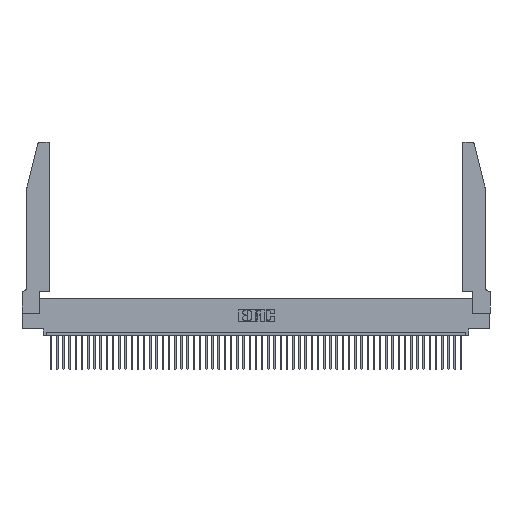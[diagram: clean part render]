
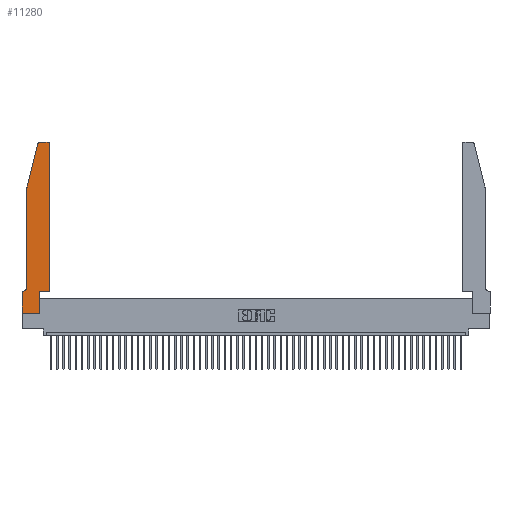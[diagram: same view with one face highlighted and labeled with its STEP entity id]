
A CAD part, top view. The second image highlights one B-rep face of the part: STEP entity #11280.
In plain terms, the highlighted planar face has unit normal (0, 0, 1).
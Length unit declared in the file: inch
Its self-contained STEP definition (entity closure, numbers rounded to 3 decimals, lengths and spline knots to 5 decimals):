
#703 = DIRECTION ( 'NONE',  ( -1., 0., 0. ) ) ;
#1174 = CARTESIAN_POINT ( 'NONE',  ( 0., 0., 0.37 ) ) ;
#1199 = DIRECTION ( 'NONE',  ( 0., 0., 1. ) ) ;
#2062 = CARTESIAN_POINT ( 'NONE',  ( 0.4205, 2.75, 0.37 ) ) ;
#2794 = DIRECTION ( 'NONE',  ( 0., 0., -1. ) ) ;
#3361 = LINE ( 'NONE', #31498, #33414 ) ;
#3362 = CARTESIAN_POINT ( 'NONE',  ( 0.0755, 0.42, 0.37 ) ) ;
#5062 = CARTESIAN_POINT ( 'NONE',  ( 0.0755, 0.35, 0.37 ) ) ;
#5239 = AXIS2_PLACEMENT_3D ( 'NONE', #48911, #1199, #17721 ) ;
#5340 = CARTESIAN_POINT ( 'NONE',  ( 0.2865, 0., 0.37 ) ) ;
#5935 = EDGE_CURVE ( 'NONE', #38857, #20977, #15634, .T. ) ;
#5965 = VECTOR ( 'NONE', #21502, 39.37008 ) ;
#6009 = VERTEX_POINT ( 'NONE', #2062 ) ;
#6143 = CARTESIAN_POINT ( 'NONE',  ( 0.4505, 0.35, 0.37 ) ) ;
#6474 = ORIENTED_EDGE ( 'NONE', *, *, #27926, .T. ) ;
#6939 = EDGE_CURVE ( 'NONE', #16477, #45572, #27984, .T. ) ;
#7575 = LINE ( 'NONE', #18554, #35811 ) ;
#8052 = AXIS2_PLACEMENT_3D ( 'NONE', #14729, #2794, #30981 ) ;
#8343 = ORIENTED_EDGE ( 'NONE', *, *, #14810, .T. ) ;
#8466 = VECTOR ( 'NONE', #29494, 39.37008 ) ;
#9025 = LINE ( 'NONE', #36225, #33503 ) ;
#9367 = ORIENTED_EDGE ( 'NONE', *, *, #30261, .T. ) ;
#9825 = VECTOR ( 'NONE', #703, 39.37008 ) ;
#9875 = DIRECTION ( 'NONE',  ( -0.239, -0.971, 0. ) ) ;
#11235 = EDGE_CURVE ( 'NONE', #22275, #40894, #43234, .T. ) ;
#11280 = ADVANCED_FACE ( 'NONE', ( #45057 ), #34998, .T. ) ;
#11444 = DIRECTION ( 'NONE',  ( 1., 0., 0. ) ) ;
#12366 = VECTOR ( 'NONE', #26677, 39.37008 ) ;
#12925 = ORIENTED_EDGE ( 'NONE', *, *, #33495, .T. ) ;
#13820 = CARTESIAN_POINT ( 'NONE',  ( 0.25487, 2.72718, 0.37 ) ) ;
#14729 = CARTESIAN_POINT ( 'NONE',  ( 0.0055, 0.42, 0.37 ) ) ;
#14810 = EDGE_CURVE ( 'NONE', #25045, #32770, #32153, .T. ) ;
#15125 = ORIENTED_EDGE ( 'NONE', *, *, #45110, .T. ) ;
#15448 = EDGE_LOOP ( 'NONE', ( #34665, #31948, #30750, #25548, #12925, #29665, #8343, #9367, #36542, #39624, #15125, #6474 ) ) ;
#15634 = LINE ( 'NONE', #25962, #12366 ) ;
#15923 = VECTOR ( 'NONE', #33576, 39.37008 ) ;
#15994 = VERTEX_POINT ( 'NONE', #5340 ) ;
#16477 = VERTEX_POINT ( 'NONE', #27066 ) ;
#16539 = LINE ( 'NONE', #33916, #27148 ) ;
#17721 = DIRECTION ( 'NONE',  ( 1., 0., 0. ) ) ;
#18554 = CARTESIAN_POINT ( 'NONE',  ( 0.4505, 0.35, 0.37 ) ) ;
#19775 = EDGE_CURVE ( 'NONE', #36288, #25045, #36807, .T. ) ;
#20473 = CARTESIAN_POINT ( 'NONE',  ( 0.4505, 2.72, 0.37 ) ) ;
#20977 = VERTEX_POINT ( 'NONE', #3362 ) ;
#21502 = DIRECTION ( 'NONE',  ( 1., 0., 0. ) ) ;
#21744 = LINE ( 'NONE', #48995, #8466 ) ;
#22275 = VERTEX_POINT ( 'NONE', #31115 ) ;
#24320 = DIRECTION ( 'NONE',  ( -1., 0., 0. ) ) ;
#25045 = VERTEX_POINT ( 'NONE', #47745 ) ;
#25548 = ORIENTED_EDGE ( 'NONE', *, *, #5935, .T. ) ;
#25962 = CARTESIAN_POINT ( 'NONE',  ( 0.0755, 2., 0.37 ) ) ;
#26677 = DIRECTION ( 'NONE',  ( 0., -1., 0. ) ) ;
#27066 = CARTESIAN_POINT ( 'NONE',  ( 0.2865, 0.35, 0.37 ) ) ;
#27148 = VECTOR ( 'NONE', #9875, 39.37008 ) ;
#27926 = EDGE_CURVE ( 'NONE', #42058, #6009, #36546, .T. ) ;
#27984 = LINE ( 'NONE', #6143, #5965 ) ;
#29494 = DIRECTION ( 'NONE',  ( 0., 1., 0. ) ) ;
#29665 = ORIENTED_EDGE ( 'NONE', *, *, #19775, .T. ) ;
#30261 = EDGE_CURVE ( 'NONE', #32770, #15994, #3361, .T. ) ;
#30750 = ORIENTED_EDGE ( 'NONE', *, *, #37956, .T. ) ;
#30981 = DIRECTION ( 'NONE',  ( -1., 0., 0. ) ) ;
#31115 = CARTESIAN_POINT ( 'NONE',  ( 0.284, 2.75, 0.37 ) ) ;
#31254 = DIRECTION ( 'NONE',  ( 0., 0., 1. ) ) ;
#31498 = CARTESIAN_POINT ( 'NONE',  ( 0., 0., 0.37 ) ) ;
#31685 = CARTESIAN_POINT ( 'NONE',  ( 0.0055, 0.35, 0.37 ) ) ;
#31948 = ORIENTED_EDGE ( 'NONE', *, *, #11235, .T. ) ;
#32153 = LINE ( 'NONE', #1174, #15923 ) ;
#32770 = VERTEX_POINT ( 'NONE', #45892 ) ;
#33414 = VECTOR ( 'NONE', #39759, 39.37008 ) ;
#33495 = EDGE_CURVE ( 'NONE', #20977, #36288, #37535, .T. ) ;
#33503 = VECTOR ( 'NONE', #24320, 39.37008 ) ;
#33576 = DIRECTION ( 'NONE',  ( 0., -1., 0. ) ) ;
#33916 = CARTESIAN_POINT ( 'NONE',  ( 0.0755, 2., 0.37 ) ) ;
#34398 = CARTESIAN_POINT ( 'NONE',  ( 0.0755, 2., 0.37 ) ) ;
#34665 = ORIENTED_EDGE ( 'NONE', *, *, #42118, .T. ) ;
#34671 = EDGE_CURVE ( 'NONE', #15994, #16477, #21744, .T. ) ;
#34998 = PLANE ( 'NONE',  #47022 ) ;
#35484 = CARTESIAN_POINT ( 'NONE',  ( 0.4205, 2.72, 0.37 ) ) ;
#35811 = VECTOR ( 'NONE', #46597, 39.37008 ) ;
#36225 = CARTESIAN_POINT ( 'NONE',  ( 0.2605, 2.75, 0.37 ) ) ;
#36288 = VERTEX_POINT ( 'NONE', #31685 ) ;
#36542 = ORIENTED_EDGE ( 'NONE', *, *, #34671, .T. ) ;
#36546 = CIRCLE ( 'NONE', #51007, 0.03 ) ;
#36807 = LINE ( 'NONE', #5062, #9825 ) ;
#37535 = CIRCLE ( 'NONE', #8052, 0.07 ) ;
#37956 = EDGE_CURVE ( 'NONE', #40894, #38857, #16539, .T. ) ;
#38081 = CARTESIAN_POINT ( 'NONE',  ( 0.4505, 0.35, 0.37 ) ) ;
#38857 = VERTEX_POINT ( 'NONE', #34398 ) ;
#39624 = ORIENTED_EDGE ( 'NONE', *, *, #6939, .T. ) ;
#39759 = DIRECTION ( 'NONE',  ( 1., 0., 0. ) ) ;
#40894 = VERTEX_POINT ( 'NONE', #13820 ) ;
#42058 = VERTEX_POINT ( 'NONE', #20473 ) ;
#42060 = DIRECTION ( 'NONE',  ( 1., 0., 0. ) ) ;
#42118 = EDGE_CURVE ( 'NONE', #6009, #22275, #9025, .T. ) ;
#43234 = CIRCLE ( 'NONE', #5239, 0.03 ) ;
#45057 = FACE_OUTER_BOUND ( 'NONE', #15448, .T. ) ;
#45110 = EDGE_CURVE ( 'NONE', #45572, #42058, #7575, .T. ) ;
#45572 = VERTEX_POINT ( 'NONE', #38081 ) ;
#45892 = CARTESIAN_POINT ( 'NONE',  ( 0., 0., 0.37 ) ) ;
#46597 = DIRECTION ( 'NONE',  ( 0., 1., 0. ) ) ;
#47022 = AXIS2_PLACEMENT_3D ( 'NONE', #51424, #48035, #42060 ) ;
#47745 = CARTESIAN_POINT ( 'NONE',  ( 0., 0.35, 0.37 ) ) ;
#48035 = DIRECTION ( 'NONE',  ( 0., 0., 1. ) ) ;
#48911 = CARTESIAN_POINT ( 'NONE',  ( 0.284, 2.72, 0.37 ) ) ;
#48995 = CARTESIAN_POINT ( 'NONE',  ( 0.2865, 0.35, 0.37 ) ) ;
#51007 = AXIS2_PLACEMENT_3D ( 'NONE', #35484, #31254, #11444 ) ;
#51424 = CARTESIAN_POINT ( 'NONE',  ( 0., 0.35, 0.37 ) ) ;
